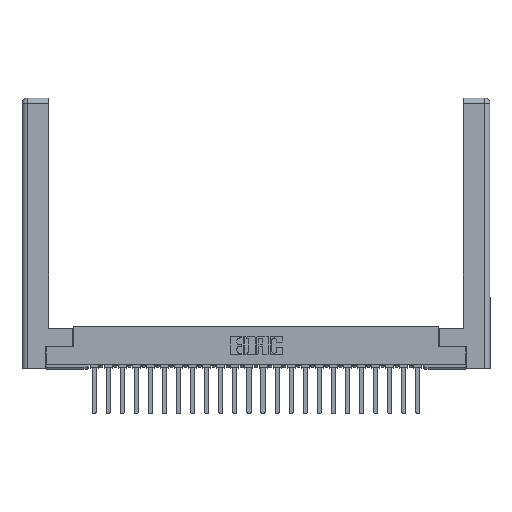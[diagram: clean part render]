
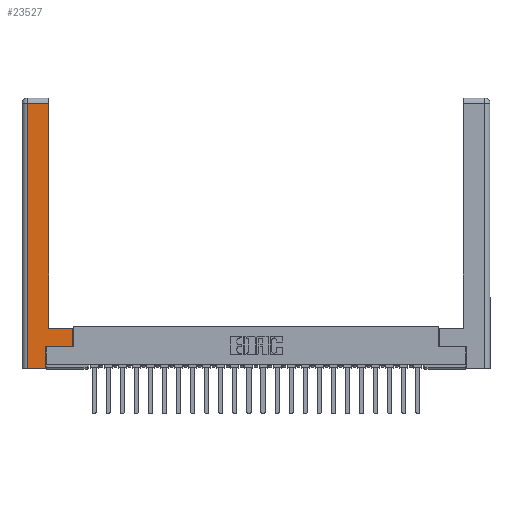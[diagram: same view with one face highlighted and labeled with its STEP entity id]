
A CAD part, top view. The second image highlights one B-rep face of the part: STEP entity #23527.
In plain terms, the highlighted planar face has unit normal (0, 0, 1).
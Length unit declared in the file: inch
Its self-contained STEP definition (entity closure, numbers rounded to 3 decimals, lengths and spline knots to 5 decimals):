
#217 = VECTOR ( 'NONE', #3334, 39.37008 ) ;
#300 = VECTOR ( 'NONE', #2131, 39.37008 ) ;
#1166 = VECTOR ( 'NONE', #16066, 39.37008 ) ;
#1195 = LINE ( 'NONE', #15465, #20613 ) ;
#1533 = CARTESIAN_POINT ( 'NONE',  ( 0.295, 2.94, 0. ) ) ;
#1543 = ORIENTED_EDGE ( 'NONE', *, *, #3460, .T. ) ;
#1753 = LINE ( 'NONE', #19757, #300 ) ;
#1833 = EDGE_CURVE ( 'NONE', #15263, #16291, #6960, .T. ) ;
#2131 = DIRECTION ( 'NONE',  ( 1., 0., 0. ) ) ;
#2627 = AXIS2_PLACEMENT_3D ( 'NONE', #5148, #8857, #21286 ) ;
#2777 = ORIENTED_EDGE ( 'NONE', *, *, #13482, .T. ) ;
#3161 = LINE ( 'NONE', #9130, #15952 ) ;
#3263 = VERTEX_POINT ( 'NONE', #23593 ) ;
#3334 = DIRECTION ( 'NONE',  ( 0., 1., 0. ) ) ;
#3460 = EDGE_CURVE ( 'NONE', #16291, #22921, #1753, .T. ) ;
#3652 = VERTEX_POINT ( 'NONE', #5431 ) ;
#4873 = FACE_OUTER_BOUND ( 'NONE', #15724, .T. ) ;
#5148 = CARTESIAN_POINT ( 'NONE',  ( 0., 0., 0. ) ) ;
#5431 = CARTESIAN_POINT ( 'NONE',  ( 0.565, 0.245, 0. ) ) ;
#6385 = CARTESIAN_POINT ( 'NONE',  ( 0.265, 0., 0. ) ) ;
#6960 = LINE ( 'NONE', #8952, #22428 ) ;
#7307 = CARTESIAN_POINT ( 'NONE',  ( 0.265, 0.245, 0. ) ) ;
#7406 = ORIENTED_EDGE ( 'NONE', *, *, #15580, .T. ) ;
#8474 = EDGE_CURVE ( 'NONE', #3652, #3263, #10727, .T. ) ;
#8857 = DIRECTION ( 'NONE',  ( 0., 0., -1. ) ) ;
#8952 = CARTESIAN_POINT ( 'NONE',  ( 0.0615, 0., 0. ) ) ;
#9130 = CARTESIAN_POINT ( 'NONE',  ( 0.295, 3., 0. ) ) ;
#9390 = DIRECTION ( 'NONE',  ( 0., 1., 0. ) ) ;
#9414 = LINE ( 'NONE', #7307, #217 ) ;
#10727 = LINE ( 'NONE', #18790, #13631 ) ;
#11331 = VERTEX_POINT ( 'NONE', #1533 ) ;
#11477 = CARTESIAN_POINT ( 'NONE',  ( 0.0615, 2.94, 0. ) ) ;
#12960 = PLANE ( 'NONE',  #2627 ) ;
#13482 = EDGE_CURVE ( 'NONE', #22921, #20777, #9414, .T. ) ;
#13631 = VECTOR ( 'NONE', #25013, 39.37008 ) ;
#15062 = EDGE_CURVE ( 'NONE', #20777, #3652, #25908, .T. ) ;
#15263 = VERTEX_POINT ( 'NONE', #19960 ) ;
#15419 = LINE ( 'NONE', #11477, #1166 ) ;
#15465 = CARTESIAN_POINT ( 'NONE',  ( 0.295, 0.45, 0. ) ) ;
#15580 = EDGE_CURVE ( 'NONE', #11331, #15263, #15419, .T. ) ;
#15724 = EDGE_LOOP ( 'NONE', ( #21600, #7406, #18781, #1543, #2777, #16586, #19982, #21773 ) ) ;
#15907 = VECTOR ( 'NONE', #21549, 39.37008 ) ;
#15952 = VECTOR ( 'NONE', #9390, 39.37008 ) ;
#16066 = DIRECTION ( 'NONE',  ( -1., 0., 0. ) ) ;
#16291 = VERTEX_POINT ( 'NONE', #17717 ) ;
#16446 = VERTEX_POINT ( 'NONE', #21419 ) ;
#16586 = ORIENTED_EDGE ( 'NONE', *, *, #15062, .T. ) ;
#17578 = CARTESIAN_POINT ( 'NONE',  ( 0.565, 0.245, 0. ) ) ;
#17717 = CARTESIAN_POINT ( 'NONE',  ( 0.0615, 0., 0. ) ) ;
#18781 = ORIENTED_EDGE ( 'NONE', *, *, #1833, .T. ) ;
#18790 = CARTESIAN_POINT ( 'NONE',  ( 0.565, 0.45, 0. ) ) ;
#18983 = CARTESIAN_POINT ( 'NONE',  ( 0.265, 0.245, 0. ) ) ;
#19757 = CARTESIAN_POINT ( 'NONE',  ( 0.265, 0., 0. ) ) ;
#19960 = CARTESIAN_POINT ( 'NONE',  ( 0.0615, 2.94, 0. ) ) ;
#19982 = ORIENTED_EDGE ( 'NONE', *, *, #8474, .T. ) ;
#20613 = VECTOR ( 'NONE', #23550, 39.37008 ) ;
#20615 = EDGE_CURVE ( 'NONE', #16446, #11331, #3161, .T. ) ;
#20777 = VERTEX_POINT ( 'NONE', #18983 ) ;
#20855 = DIRECTION ( 'NONE',  ( 0., -1., 0. ) ) ;
#21286 = DIRECTION ( 'NONE',  ( -1., 0., 0. ) ) ;
#21419 = CARTESIAN_POINT ( 'NONE',  ( 0.295, 0.45, 0. ) ) ;
#21549 = DIRECTION ( 'NONE',  ( 1., 0., 0. ) ) ;
#21600 = ORIENTED_EDGE ( 'NONE', *, *, #20615, .T. ) ;
#21773 = ORIENTED_EDGE ( 'NONE', *, *, #21831, .T. ) ;
#21831 = EDGE_CURVE ( 'NONE', #3263, #16446, #1195, .T. ) ;
#22428 = VECTOR ( 'NONE', #20855, 39.37008 ) ;
#22921 = VERTEX_POINT ( 'NONE', #6385 ) ;
#23527 = ADVANCED_FACE ( 'NONE', ( #4873 ), #12960, .F. ) ;
#23550 = DIRECTION ( 'NONE',  ( -1., 0., 0. ) ) ;
#23593 = CARTESIAN_POINT ( 'NONE',  ( 0.565, 0.45, 0. ) ) ;
#25013 = DIRECTION ( 'NONE',  ( 0., 1., 0. ) ) ;
#25908 = LINE ( 'NONE', #17578, #15907 ) ;
